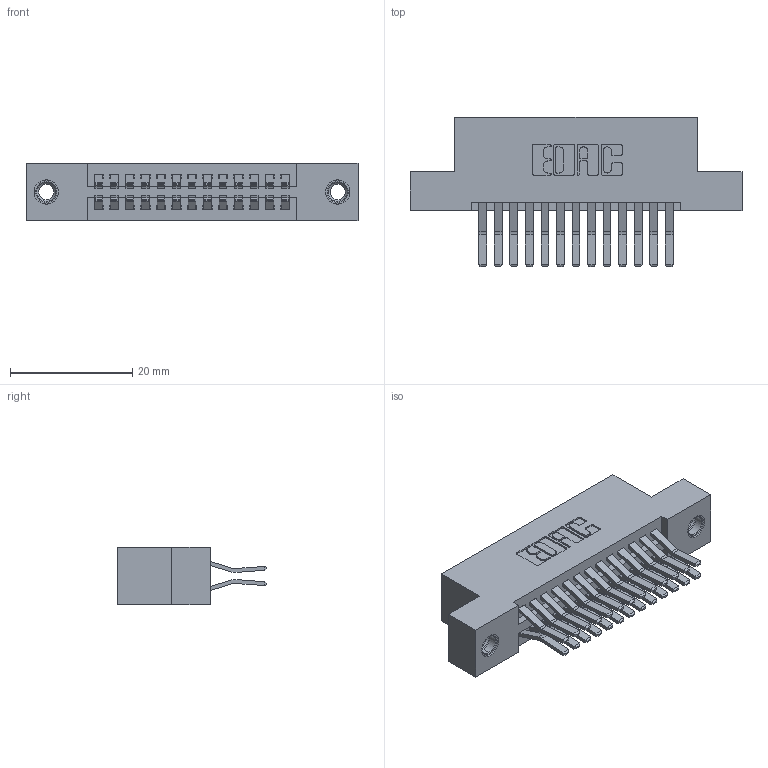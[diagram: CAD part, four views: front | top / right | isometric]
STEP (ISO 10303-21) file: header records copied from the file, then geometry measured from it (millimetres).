
FILE_DESCRIPTION (( 'STEP AP203' ), '1' );
FILE_NAME ('395-026-560-207.STEP', '2018-11-10T03:32:17', ( '' ), ( '' ), 'SwSTEP 2.0', 'SolidWorks 2016', '' );
FILE_SCHEMA (( 'CONFIG_CONTROL_DESIGN' ));
Length unit declared in the file: inch
Products named in the file (4): 395-026-560-207; 345-292-001_560 Tail; 345-250-001_345-250-005-103; 345 Part_Flush Mounting Lugs - 0.156 Dia-TI
Assembly tree (29 placements, depth 2):
  395-026-560-207
    345 Part_Flush Mounting Lugs - 0.156 Dia-TI
    345-292-001_560 Tail  x26
    345-250-001_345-250-005-103  x2
Bounding box: 54.23 x 24.45 x 9.4 mm (x, y, z)
Volume: 5155.6 mm3; surface area: 7525.3 mm2
Topology: 29 solids, 29 shells, 1538 faces, 4507 edges, 2962 vertices
Faces by surface type: plane 970, cylinder 552, cone 12, torus 4
Entity records: 15378 total; most frequent: CARTESIAN_POINT 2587, ORIENTED_EDGE 2514, DIRECTION 2347, EDGE_CURVE 1257, VECTOR 1049, LINE 1049, VERTEX_POINT 832, AXIS2_PLACEMENT_3D 649
